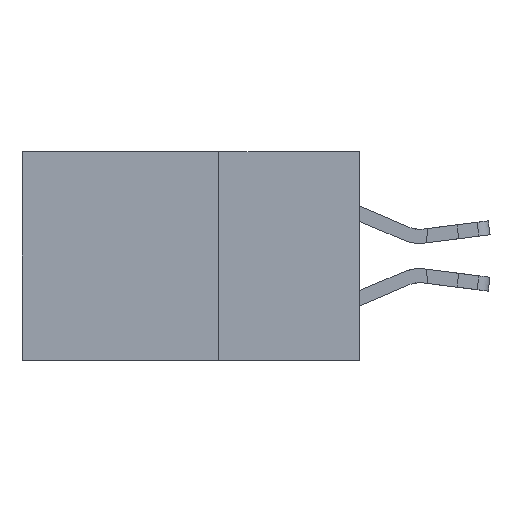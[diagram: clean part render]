
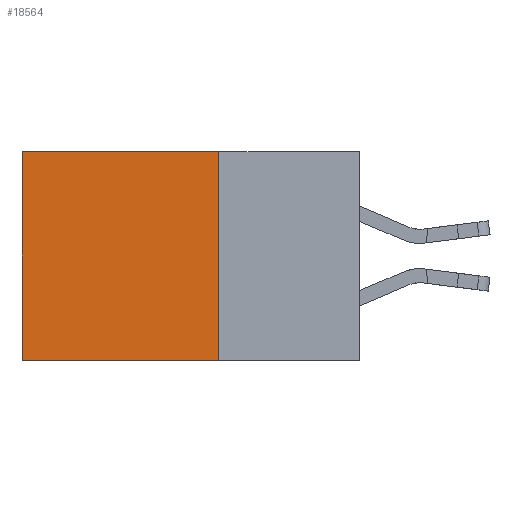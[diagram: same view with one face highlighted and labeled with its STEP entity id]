
A CAD part, left-side view. The second image highlights one B-rep face of the part: STEP entity #18564.
In plain terms, the highlighted planar face has unit normal (-1, 0, 0).
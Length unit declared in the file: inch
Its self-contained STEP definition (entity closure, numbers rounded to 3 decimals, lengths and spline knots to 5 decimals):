
#1025 = AXIS2_PLACEMENT_3D ( 'NONE', #8471, #23188, #1200 ) ;
#1200 = DIRECTION ( 'NONE',  ( 0., 0., -1. ) ) ;
#1801 = ORIENTED_EDGE ( 'NONE', *, *, #12583, .F. ) ;
#2775 = FACE_OUTER_BOUND ( 'NONE', #9231, .T. ) ;
#4135 = CARTESIAN_POINT ( 'NONE',  ( 0.2875, 0.6, 0. ) ) ;
#4140 = LINE ( 'NONE', #22379, #22407 ) ;
#5470 = EDGE_CURVE ( 'NONE', #23195, #21370, #6692, .T. ) ;
#6692 = LINE ( 'NONE', #14104, #12410 ) ;
#7396 = EDGE_CURVE ( 'NONE', #15416, #16774, #15714, .T. ) ;
#8471 = CARTESIAN_POINT ( 'NONE',  ( 0.2875, 0.25, 0. ) ) ;
#8955 = ORIENTED_EDGE ( 'NONE', *, *, #5470, .T. ) ;
#9231 = EDGE_LOOP ( 'NONE', ( #8955, #1801, #9777, #15856 ) ) ;
#9777 = ORIENTED_EDGE ( 'NONE', *, *, #7396, .F. ) ;
#11888 = CARTESIAN_POINT ( 'NONE',  ( 0.2875, 0.25, -0.37 ) ) ;
#12410 = VECTOR ( 'NONE', #16042, 39.37008 ) ;
#12583 = EDGE_CURVE ( 'NONE', #16774, #21370, #15630, .T. ) ;
#13126 = DIRECTION ( 'NONE',  ( 0., 1., 0. ) ) ;
#13264 = CARTESIAN_POINT ( 'NONE',  ( 0.2875, 0.25, 0. ) ) ;
#13511 = CARTESIAN_POINT ( 'NONE',  ( 0.2875, 0.25, -0.37 ) ) ;
#13744 = CARTESIAN_POINT ( 'NONE',  ( 0.2875, 0.6, -0.37 ) ) ;
#14104 = CARTESIAN_POINT ( 'NONE',  ( 0.2875, 0.6, 0. ) ) ;
#14213 = VECTOR ( 'NONE', #21470, 39.37008 ) ;
#15164 = DIRECTION ( 'NONE',  ( 0., 0., -1. ) ) ;
#15416 = VERTEX_POINT ( 'NONE', #13264 ) ;
#15630 = LINE ( 'NONE', #11888, #14213 ) ;
#15714 = LINE ( 'NONE', #22699, #20667 ) ;
#15856 = ORIENTED_EDGE ( 'NONE', *, *, #19693, .T. ) ;
#16042 = DIRECTION ( 'NONE',  ( 0., 0., -1. ) ) ;
#16774 = VERTEX_POINT ( 'NONE', #13511 ) ;
#18564 = ADVANCED_FACE ( 'NONE', ( #2775 ), #21357, .F. ) ;
#19693 = EDGE_CURVE ( 'NONE', #15416, #23195, #4140, .T. ) ;
#20667 = VECTOR ( 'NONE', #15164, 39.37008 ) ;
#21357 = PLANE ( 'NONE',  #1025 ) ;
#21370 = VERTEX_POINT ( 'NONE', #13744 ) ;
#21470 = DIRECTION ( 'NONE',  ( 0., 1., 0. ) ) ;
#22379 = CARTESIAN_POINT ( 'NONE',  ( 0.2875, 0.25, 0. ) ) ;
#22407 = VECTOR ( 'NONE', #13126, 39.37008 ) ;
#22699 = CARTESIAN_POINT ( 'NONE',  ( 0.2875, 0.25, 0. ) ) ;
#23188 = DIRECTION ( 'NONE',  ( 1., 0., 0. ) ) ;
#23195 = VERTEX_POINT ( 'NONE', #4135 ) ;
